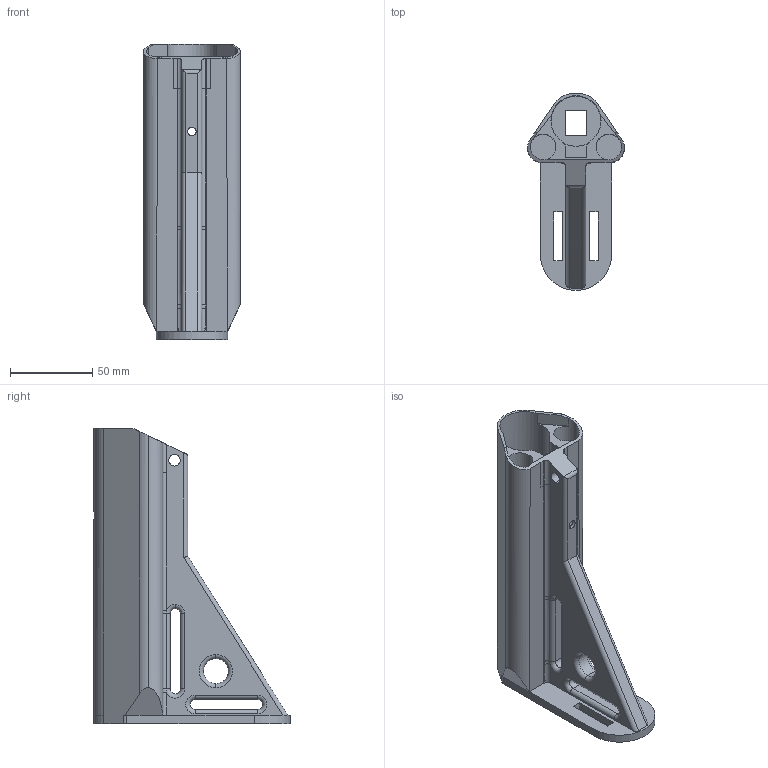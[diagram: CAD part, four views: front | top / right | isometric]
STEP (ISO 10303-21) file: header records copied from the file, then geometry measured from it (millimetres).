
FILE_DESCRIPTION (( 'STEP AP214' ), '1' );
FILE_NAME ('Sopmod Stock.STEP', '2013-06-18T15:25:11', ( 'Asher' ), ( '' ), 'SwSTEP 2.0', 'SolidWorks 2013', '' );
FILE_SCHEMA (( 'AUTOMOTIVE_DESIGN' ));
Length unit declared in the file: millimetre
Products named in the file (1): Sopmod Stock
Bounding box: 59 x 119.51 x 179.71 mm (x, y, z)
Volume: 177142.7 mm3; surface area: 84578.6 mm2
Topology: 1 solids, 1 shells, 149 faces, 398 edges, 252 vertices
Faces by surface type: plane 73, cylinder 56, torus 14, bspline 6
Entity records: 4920 total; most frequent: CARTESIAN_POINT 1188, ORIENTED_EDGE 796, DIRECTION 754, EDGE_CURVE 398, AXIS2_PLACEMENT_3D 260, VERTEX_POINT 252, LINE 234, VECTOR 234
